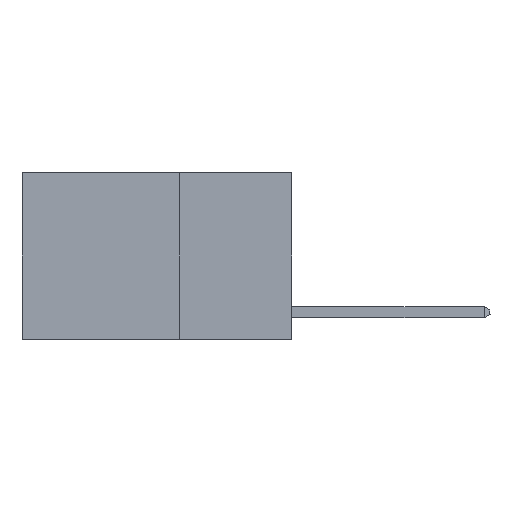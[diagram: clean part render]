
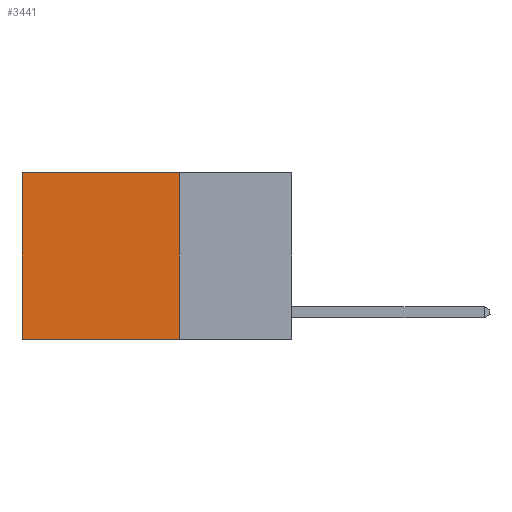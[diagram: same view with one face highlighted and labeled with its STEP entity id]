
A CAD part, left-side view. The second image highlights one B-rep face of the part: STEP entity #3441.
In plain terms, the highlighted planar face has unit normal (-1, 0, 0).
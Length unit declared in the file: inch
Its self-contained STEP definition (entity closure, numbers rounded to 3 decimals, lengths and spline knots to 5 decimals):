
#92 = DIRECTION ( 'NONE',  ( 0., 0., -1. ) ) ;
#398 = EDGE_CURVE ( 'NONE', #2058, #8384, #10327, .T. ) ;
#926 = ORIENTED_EDGE ( 'NONE', *, *, #10837, .T. ) ;
#979 = DIRECTION ( 'NONE',  ( 0., 0., -1. ) ) ;
#1094 = LINE ( 'NONE', #8466, #5081 ) ;
#1243 = LINE ( 'NONE', #5578, #8465 ) ;
#1934 = CARTESIAN_POINT ( 'NONE',  ( 0.2625, 0.25, -0.37 ) ) ;
#2058 = VERTEX_POINT ( 'NONE', #10386 ) ;
#2709 = CARTESIAN_POINT ( 'NONE',  ( 0.2625, 0.25, -0.37 ) ) ;
#2804 = CARTESIAN_POINT ( 'NONE',  ( 0.2625, 0.25, 0. ) ) ;
#3188 = EDGE_CURVE ( 'NONE', #2058, #5657, #1243, .T. ) ;
#3360 = CARTESIAN_POINT ( 'NONE',  ( 0.2625, 0.6, -0.37 ) ) ;
#3439 = ORIENTED_EDGE ( 'NONE', *, *, #398, .F. ) ;
#3441 = ADVANCED_FACE ( 'NONE', ( #10648 ), #7157, .F. ) ;
#3781 = EDGE_CURVE ( 'NONE', #8384, #7338, #9520, .T. ) ;
#3954 = CARTESIAN_POINT ( 'NONE',  ( 0.2625, 0.6, 0. ) ) ;
#4245 = VECTOR ( 'NONE', #92, 39.37008 ) ;
#4747 = DIRECTION ( 'NONE',  ( 1., 0., 0. ) ) ;
#5081 = VECTOR ( 'NONE', #979, 39.37008 ) ;
#5578 = CARTESIAN_POINT ( 'NONE',  ( 0.2625, 0.25, 0. ) ) ;
#5657 = VERTEX_POINT ( 'NONE', #3954 ) ;
#5993 = EDGE_LOOP ( 'NONE', ( #926, #9633, #3439, #9099 ) ) ;
#6641 = AXIS2_PLACEMENT_3D ( 'NONE', #8006, #4747, #7103 ) ;
#6708 = DIRECTION ( 'NONE',  ( 0., 1., 0. ) ) ;
#7103 = DIRECTION ( 'NONE',  ( 0., 0., -1. ) ) ;
#7157 = PLANE ( 'NONE',  #6641 ) ;
#7338 = VERTEX_POINT ( 'NONE', #3360 ) ;
#8006 = CARTESIAN_POINT ( 'NONE',  ( 0.2625, 0.25, 0. ) ) ;
#8384 = VERTEX_POINT ( 'NONE', #2709 ) ;
#8465 = VECTOR ( 'NONE', #8819, 39.37008 ) ;
#8466 = CARTESIAN_POINT ( 'NONE',  ( 0.2625, 0.6, 0. ) ) ;
#8819 = DIRECTION ( 'NONE',  ( 0., 1., 0. ) ) ;
#9099 = ORIENTED_EDGE ( 'NONE', *, *, #3188, .T. ) ;
#9520 = LINE ( 'NONE', #1934, #10594 ) ;
#9633 = ORIENTED_EDGE ( 'NONE', *, *, #3781, .F. ) ;
#10327 = LINE ( 'NONE', #2804, #4245 ) ;
#10386 = CARTESIAN_POINT ( 'NONE',  ( 0.2625, 0.25, 0. ) ) ;
#10594 = VECTOR ( 'NONE', #6708, 39.37008 ) ;
#10648 = FACE_OUTER_BOUND ( 'NONE', #5993, .T. ) ;
#10837 = EDGE_CURVE ( 'NONE', #5657, #7338, #1094, .T. ) ;
